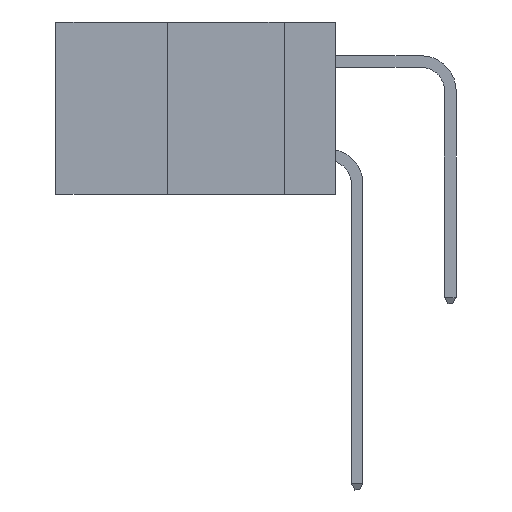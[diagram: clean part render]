
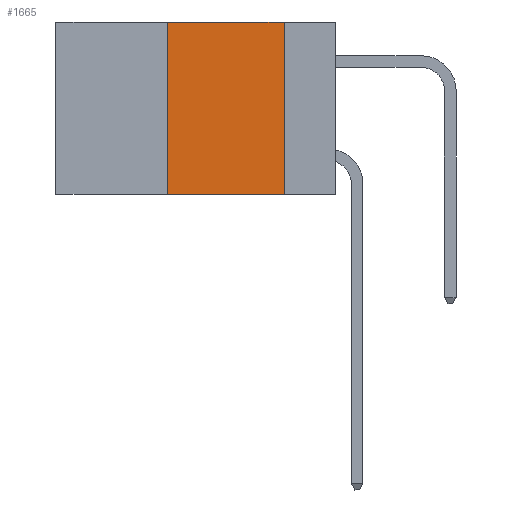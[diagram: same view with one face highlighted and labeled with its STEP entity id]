
A CAD part, left-side view. The second image highlights one B-rep face of the part: STEP entity #1665.
In plain terms, the highlighted planar face has unit normal (-1, 0, 0).
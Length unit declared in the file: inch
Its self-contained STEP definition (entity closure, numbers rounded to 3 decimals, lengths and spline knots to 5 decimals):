
#316 = CARTESIAN_POINT ( 'NONE',  ( 0., 0.6, 0. ) ) ;
#337 = CARTESIAN_POINT ( 'NONE',  ( 0., 0.36, 0. ) ) ;
#532 = VERTEX_POINT ( 'NONE', #5996 ) ;
#558 = ORIENTED_EDGE ( 'NONE', *, *, #11323, .F. ) ;
#768 = VERTEX_POINT ( 'NONE', #3884 ) ;
#1665 = ADVANCED_FACE ( 'NONE', ( #5310 ), #9495, .F. ) ;
#1969 = LINE ( 'NONE', #4250, #6627 ) ;
#2232 = VECTOR ( 'NONE', #9360, 39.37008 ) ;
#2713 = LINE ( 'NONE', #337, #9706 ) ;
#3214 = ORIENTED_EDGE ( 'NONE', *, *, #7692, .F. ) ;
#3498 = ORIENTED_EDGE ( 'NONE', *, *, #5913, .T. ) ;
#3765 = VERTEX_POINT ( 'NONE', #9078 ) ;
#3884 = CARTESIAN_POINT ( 'NONE',  ( 0., 0.11, -0.37 ) ) ;
#4060 = VERTEX_POINT ( 'NONE', #8545 ) ;
#4250 = CARTESIAN_POINT ( 'NONE',  ( 0., 0.6, -0.37 ) ) ;
#4265 = DIRECTION ( 'NONE',  ( 0., -1., 0. ) ) ;
#5303 = DIRECTION ( 'NONE',  ( 0., -1., 0. ) ) ;
#5310 = FACE_OUTER_BOUND ( 'NONE', #11074, .T. ) ;
#5665 = AXIS2_PLACEMENT_3D ( 'NONE', #10416, #9837, #5938 ) ;
#5913 = EDGE_CURVE ( 'NONE', #3765, #768, #1969, .T. ) ;
#5938 = DIRECTION ( 'NONE',  ( 0., 0., -1. ) ) ;
#5996 = CARTESIAN_POINT ( 'NONE',  ( 0., 0.11, 0. ) ) ;
#6049 = DIRECTION ( 'NONE',  ( 0., 0., 1. ) ) ;
#6381 = VECTOR ( 'NONE', #4265, 39.37008 ) ;
#6627 = VECTOR ( 'NONE', #5303, 39.37008 ) ;
#7413 = LINE ( 'NONE', #11213, #2232 ) ;
#7692 = EDGE_CURVE ( 'NONE', #3765, #4060, #2713, .T. ) ;
#8284 = EDGE_CURVE ( 'NONE', #532, #768, #7413, .T. ) ;
#8545 = CARTESIAN_POINT ( 'NONE',  ( 0., 0.36, 0. ) ) ;
#8730 = LINE ( 'NONE', #316, #6381 ) ;
#9078 = CARTESIAN_POINT ( 'NONE',  ( 0., 0.36, -0.37 ) ) ;
#9360 = DIRECTION ( 'NONE',  ( 0., 0., -1. ) ) ;
#9495 = PLANE ( 'NONE',  #5665 ) ;
#9706 = VECTOR ( 'NONE', #6049, 39.37008 ) ;
#9837 = DIRECTION ( 'NONE',  ( 1., 0., 0. ) ) ;
#10188 = ORIENTED_EDGE ( 'NONE', *, *, #8284, .F. ) ;
#10416 = CARTESIAN_POINT ( 'NONE',  ( 0., 0.6, 0. ) ) ;
#11074 = EDGE_LOOP ( 'NONE', ( #10188, #558, #3214, #3498 ) ) ;
#11213 = CARTESIAN_POINT ( 'NONE',  ( 0., 0.11, 0. ) ) ;
#11323 = EDGE_CURVE ( 'NONE', #4060, #532, #8730, .T. ) ;
